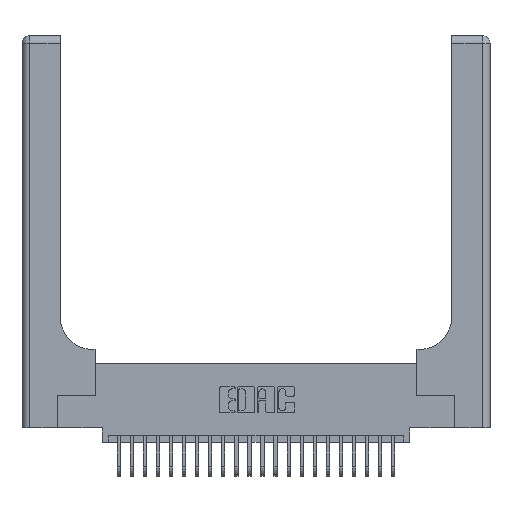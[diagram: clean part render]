
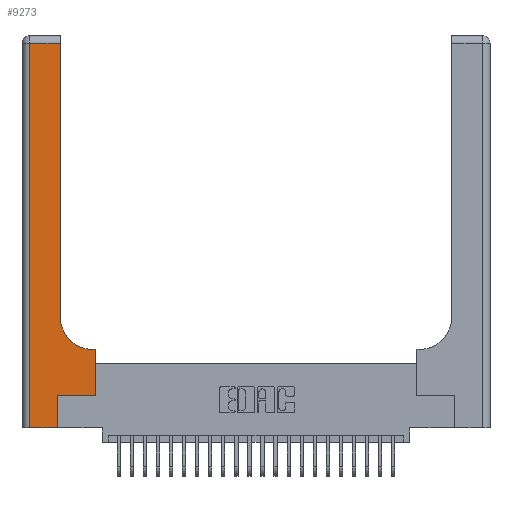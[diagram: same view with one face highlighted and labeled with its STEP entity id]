
A CAD part, top view. The second image highlights one B-rep face of the part: STEP entity #9273.
In plain terms, the highlighted planar face has unit normal (0, 0, 1).
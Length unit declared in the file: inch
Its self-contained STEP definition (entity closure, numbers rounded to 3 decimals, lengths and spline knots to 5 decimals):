
#619 = VECTOR ( 'NONE', #23865, 39.37008 ) ;
#822 = CARTESIAN_POINT ( 'NONE',  ( 0.2915, 0.85, 0.37 ) ) ;
#1841 = VERTEX_POINT ( 'NONE', #19637 ) ;
#1883 = VERTEX_POINT ( 'NONE', #822 ) ;
#2033 = VERTEX_POINT ( 'NONE', #22315 ) ;
#2560 = CARTESIAN_POINT ( 'NONE',  ( 0., 3., 0.37 ) ) ;
#2734 = EDGE_CURVE ( 'NONE', #16238, #7617, #13273, .T. ) ;
#2947 = VECTOR ( 'NONE', #21730, 39.37008 ) ;
#4158 = AXIS2_PLACEMENT_3D ( 'NONE', #2560, #19792, #8397 ) ;
#5262 = ORIENTED_EDGE ( 'NONE', *, *, #9740, .T. ) ;
#6157 = ORIENTED_EDGE ( 'NONE', *, *, #10694, .T. ) ;
#6412 = VECTOR ( 'NONE', #8691, 39.37008 ) ;
#6451 = PLANE ( 'NONE',  #4158 ) ;
#6708 = VECTOR ( 'NONE', #16842, 39.37008 ) ;
#6717 = ORIENTED_EDGE ( 'NONE', *, *, #10874, .T. ) ;
#6740 = CARTESIAN_POINT ( 'NONE',  ( 0.5585, 0.25, 0.37 ) ) ;
#7311 = CARTESIAN_POINT ( 'NONE',  ( 0.06, 3., 0.37 ) ) ;
#7598 = CARTESIAN_POINT ( 'NONE',  ( 0.2915, 0.6, 0.37 ) ) ;
#7617 = VERTEX_POINT ( 'NONE', #10789 ) ;
#8210 = CARTESIAN_POINT ( 'NONE',  ( 0.5415, 0.85, 0.37 ) ) ;
#8220 = EDGE_CURVE ( 'NONE', #1841, #2033, #10879, .T. ) ;
#8397 = DIRECTION ( 'NONE',  ( -1., 0., 0. ) ) ;
#8419 = FACE_OUTER_BOUND ( 'NONE', #17592, .T. ) ;
#8691 = DIRECTION ( 'NONE',  ( 0., 1., 0. ) ) ;
#9051 = CARTESIAN_POINT ( 'NONE',  ( 0.06, 0., 0.37 ) ) ;
#9273 = ADVANCED_FACE ( 'NONE', ( #8419 ), #6451, .F. ) ;
#9548 = DIRECTION ( 'NONE',  ( -1., 0., 0. ) ) ;
#9740 = EDGE_CURVE ( 'NONE', #21590, #23677, #13651, .T. ) ;
#10115 = ORIENTED_EDGE ( 'NONE', *, *, #14828, .T. ) ;
#10152 = DIRECTION ( 'NONE',  ( 1., 0., 0. ) ) ;
#10159 = ORIENTED_EDGE ( 'NONE', *, *, #24419, .T. ) ;
#10204 = CARTESIAN_POINT ( 'NONE',  ( 0., 0., 0.37 ) ) ;
#10479 = EDGE_CURVE ( 'NONE', #2033, #16238, #22164, .T. ) ;
#10597 = CARTESIAN_POINT ( 'NONE',  ( 0.269, 0.25, 0.37 ) ) ;
#10694 = EDGE_CURVE ( 'NONE', #23677, #16224, #11802, .T. ) ;
#10789 = CARTESIAN_POINT ( 'NONE',  ( 0.5415, 0.6, 0.37 ) ) ;
#10874 = EDGE_CURVE ( 'NONE', #1883, #21590, #17740, .T. ) ;
#10879 = LINE ( 'NONE', #10597, #619 ) ;
#11425 = ORIENTED_EDGE ( 'NONE', *, *, #8220, .T. ) ;
#11624 = EDGE_CURVE ( 'NONE', #7617, #1883, #21242, .T. ) ;
#11802 = LINE ( 'NONE', #7311, #6708 ) ;
#12099 = DIRECTION ( 'NONE',  ( 1., 0., 0. ) ) ;
#12307 = CARTESIAN_POINT ( 'NONE',  ( 0.269, 0., 0.37 ) ) ;
#12405 = CARTESIAN_POINT ( 'NONE',  ( 0.269, 0., 0.37 ) ) ;
#12538 = LINE ( 'NONE', #10204, #21975 ) ;
#12703 = ORIENTED_EDGE ( 'NONE', *, *, #10479, .T. ) ;
#13273 = LINE ( 'NONE', #7598, #22706 ) ;
#13596 = DIRECTION ( 'NONE',  ( 0., 1., 0. ) ) ;
#13651 = LINE ( 'NONE', #19268, #18674 ) ;
#13997 = VERTEX_POINT ( 'NONE', #12405 ) ;
#14697 = ORIENTED_EDGE ( 'NONE', *, *, #2734, .T. ) ;
#14774 = CARTESIAN_POINT ( 'NONE',  ( 0.5585, 0.6, 0.37 ) ) ;
#14828 = EDGE_CURVE ( 'NONE', #16224, #13997, #12538, .T. ) ;
#15526 = ORIENTED_EDGE ( 'NONE', *, *, #11624, .T. ) ;
#16224 = VERTEX_POINT ( 'NONE', #9051 ) ;
#16238 = VERTEX_POINT ( 'NONE', #14774 ) ;
#16842 = DIRECTION ( 'NONE',  ( 0., -1., 0. ) ) ;
#16957 = CARTESIAN_POINT ( 'NONE',  ( 0.2915, 2.94, 0.37 ) ) ;
#17155 = VECTOR ( 'NONE', #13596, 39.37008 ) ;
#17592 = EDGE_LOOP ( 'NONE', ( #6717, #5262, #6157, #10115, #10159, #11425, #12703, #14697, #15526 ) ) ;
#17632 = LINE ( 'NONE', #12307, #2947 ) ;
#17740 = LINE ( 'NONE', #22981, #17155 ) ;
#17990 = AXIS2_PLACEMENT_3D ( 'NONE', #8210, #21480, #10152 ) ;
#18674 = VECTOR ( 'NONE', #21160, 39.37008 ) ;
#19268 = CARTESIAN_POINT ( 'NONE',  ( 0., 2.94, 0.37 ) ) ;
#19637 = CARTESIAN_POINT ( 'NONE',  ( 0.269, 0.25, 0.37 ) ) ;
#19792 = DIRECTION ( 'NONE',  ( 0., 0., -1. ) ) ;
#21160 = DIRECTION ( 'NONE',  ( -1., 0., 0. ) ) ;
#21242 = CIRCLE ( 'NONE', #17990, 0.25 ) ;
#21480 = DIRECTION ( 'NONE',  ( 0., 0., -1. ) ) ;
#21590 = VERTEX_POINT ( 'NONE', #16957 ) ;
#21730 = DIRECTION ( 'NONE',  ( 0., 1., 0. ) ) ;
#21975 = VECTOR ( 'NONE', #12099, 39.37008 ) ;
#22164 = LINE ( 'NONE', #6740, #6412 ) ;
#22315 = CARTESIAN_POINT ( 'NONE',  ( 0.5585, 0.25, 0.37 ) ) ;
#22706 = VECTOR ( 'NONE', #9548, 39.37008 ) ;
#22981 = CARTESIAN_POINT ( 'NONE',  ( 0.2915, 3., 0.37 ) ) ;
#23245 = CARTESIAN_POINT ( 'NONE',  ( 0.06, 2.94, 0.37 ) ) ;
#23677 = VERTEX_POINT ( 'NONE', #23245 ) ;
#23865 = DIRECTION ( 'NONE',  ( 1., 0., 0. ) ) ;
#24419 = EDGE_CURVE ( 'NONE', #13997, #1841, #17632, .T. ) ;
